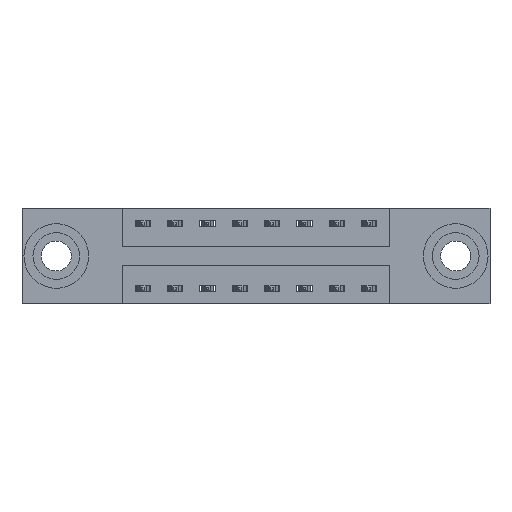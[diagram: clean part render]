
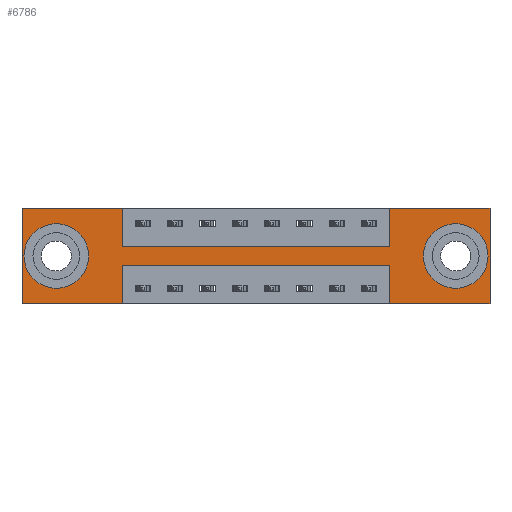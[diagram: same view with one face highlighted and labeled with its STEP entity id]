
A CAD part, front view. The second image highlights one B-rep face of the part: STEP entity #6786.
In plain terms, the highlighted planar face has unit normal (0, -1, 0).
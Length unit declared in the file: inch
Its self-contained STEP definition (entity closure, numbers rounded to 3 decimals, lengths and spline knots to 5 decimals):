
#21 = VECTOR ( 'NONE', #5674, 39.37008 ) ;
#95 = DIRECTION ( 'NONE',  ( 0., 0., 1. ) ) ;
#140 = EDGE_CURVE ( 'NONE', #5483, #7407, #8158, .T. ) ;
#218 = EDGE_CURVE ( 'NONE', #9366, #9716, #7409, .T. ) ;
#443 = FACE_BOUND ( 'NONE', #2200, .T. ) ;
#562 = AXIS2_PLACEMENT_3D ( 'NONE', #6055, #1032, #6862 ) ;
#736 = LINE ( 'NONE', #6050, #8720 ) ;
#753 = CARTESIAN_POINT ( 'NONE',  ( 0.3875, 0., 0. ) ) ;
#939 = AXIS2_PLACEMENT_3D ( 'NONE', #6089, #2746, #8485 ) ;
#1032 = DIRECTION ( 'NONE',  ( 0., 1., 0. ) ) ;
#1037 = CARTESIAN_POINT ( 'NONE',  ( 1.81, 0., 0. ) ) ;
#1053 = CARTESIAN_POINT ( 'NONE',  ( 1.4225, 0., -0.37 ) ) ;
#1063 = CARTESIAN_POINT ( 'NONE',  ( 1.81, 0., 0. ) ) ;
#1160 = ORIENTED_EDGE ( 'NONE', *, *, #9546, .F. ) ;
#1297 = CARTESIAN_POINT ( 'NONE',  ( 0.1325, 0., -0.185 ) ) ;
#1353 = ORIENTED_EDGE ( 'NONE', *, *, #4630, .T. ) ;
#1377 = DIRECTION ( 'NONE',  ( 1., 0., 0. ) ) ;
#1467 = ORIENTED_EDGE ( 'NONE', *, *, #218, .F. ) ;
#1550 = DIRECTION ( 'NONE',  ( 0., 1., 0. ) ) ;
#1577 = ORIENTED_EDGE ( 'NONE', *, *, #9678, .F. ) ;
#1593 = VECTOR ( 'NONE', #7326, 39.37008 ) ;
#1604 = DIRECTION ( 'NONE',  ( 0., 0., -1. ) ) ;
#1704 = AXIS2_PLACEMENT_3D ( 'NONE', #6538, #1550, #7331 ) ;
#1717 = EDGE_CURVE ( 'NONE', #7351, #2289, #8508, .T. ) ;
#1751 = CARTESIAN_POINT ( 'NONE',  ( 1.4225, 0., 0. ) ) ;
#1907 = LINE ( 'NONE', #4998, #10024 ) ;
#1920 = PLANE ( 'NONE',  #939 ) ;
#1961 = VERTEX_POINT ( 'NONE', #7584 ) ;
#1974 = LINE ( 'NONE', #2035, #3958 ) ;
#1984 = LINE ( 'NONE', #4860, #6172 ) ;
#1992 = EDGE_CURVE ( 'NONE', #5678, #4226, #7871, .T. ) ;
#2035 = CARTESIAN_POINT ( 'NONE',  ( 0., 0., -0.37 ) ) ;
#2075 = CIRCLE ( 'NONE', #2267, 0.078 ) ;
#2097 = DIRECTION ( 'NONE',  ( 0., 0., 1. ) ) ;
#2126 = CARTESIAN_POINT ( 'NONE',  ( 0.1325, 0., -0.107 ) ) ;
#2141 = DIRECTION ( 'NONE',  ( 0., 0., 1. ) ) ;
#2200 = EDGE_LOOP ( 'NONE', ( #7179, #1353 ) ) ;
#2224 = EDGE_CURVE ( 'NONE', #4226, #5678, #9817, .T. ) ;
#2250 = AXIS2_PLACEMENT_3D ( 'NONE', #1297, #7099, #2141 ) ;
#2267 = AXIS2_PLACEMENT_3D ( 'NONE', #7399, #2464, #8216 ) ;
#2289 = VERTEX_POINT ( 'NONE', #4767 ) ;
#2301 = CARTESIAN_POINT ( 'NONE',  ( 1.4225, 0., -0.37 ) ) ;
#2464 = DIRECTION ( 'NONE',  ( 0., 1., 0. ) ) ;
#2618 = VECTOR ( 'NONE', #1377, 39.37008 ) ;
#2663 = FACE_BOUND ( 'NONE', #4462, .T. ) ;
#2746 = DIRECTION ( 'NONE',  ( 0., -1., 0. ) ) ;
#2778 = VERTEX_POINT ( 'NONE', #3030 ) ;
#2782 = ORIENTED_EDGE ( 'NONE', *, *, #140, .F. ) ;
#2853 = VERTEX_POINT ( 'NONE', #6460 ) ;
#2868 = DIRECTION ( 'NONE',  ( -1., 0., 0. ) ) ;
#3030 = CARTESIAN_POINT ( 'NONE',  ( 0., 0., 0. ) ) ;
#3063 = CIRCLE ( 'NONE', #1704, 0.078 ) ;
#3576 = CARTESIAN_POINT ( 'NONE',  ( 0.3875, 0., -0.22 ) ) ;
#3653 = ORIENTED_EDGE ( 'NONE', *, *, #10394, .F. ) ;
#3719 = DIRECTION ( 'NONE',  ( 1., 0., 0. ) ) ;
#3753 = CARTESIAN_POINT ( 'NONE',  ( 1.6775, 0., -0.263 ) ) ;
#3958 = VECTOR ( 'NONE', #2868, 39.37008 ) ;
#4028 = ORIENTED_EDGE ( 'NONE', *, *, #9071, .F. ) ;
#4029 = VERTEX_POINT ( 'NONE', #7032 ) ;
#4053 = EDGE_CURVE ( 'NONE', #4668, #7351, #1907, .T. ) ;
#4148 = ORIENTED_EDGE ( 'NONE', *, *, #8516, .F. ) ;
#4226 = VERTEX_POINT ( 'NONE', #9182 ) ;
#4331 = VERTEX_POINT ( 'NONE', #6901 ) ;
#4399 = VERTEX_POINT ( 'NONE', #4602 ) ;
#4462 = EDGE_LOOP ( 'NONE', ( #10114, #4656 ) ) ;
#4602 = CARTESIAN_POINT ( 'NONE',  ( 1.4225, 0., -0.15 ) ) ;
#4630 = EDGE_CURVE ( 'NONE', #5597, #1961, #3063, .T. ) ;
#4656 = ORIENTED_EDGE ( 'NONE', *, *, #2224, .T. ) ;
#4668 = VERTEX_POINT ( 'NONE', #3576 ) ;
#4678 = FACE_OUTER_BOUND ( 'NONE', #5301, .T. ) ;
#4732 = EDGE_CURVE ( 'NONE', #1961, #5597, #2075, .T. ) ;
#4767 = CARTESIAN_POINT ( 'NONE',  ( 0., 0., -0.37 ) ) ;
#4781 = VECTOR ( 'NONE', #1604, 39.37008 ) ;
#4860 = CARTESIAN_POINT ( 'NONE',  ( 0.3875, 0., -0.15 ) ) ;
#4890 = LINE ( 'NONE', #9465, #2618 ) ;
#4978 = EDGE_CURVE ( 'NONE', #7407, #4668, #736, .T. ) ;
#4997 = VECTOR ( 'NONE', #95, 39.37008 ) ;
#4998 = CARTESIAN_POINT ( 'NONE',  ( 0.3875, 0., -0.37 ) ) ;
#5301 = EDGE_LOOP ( 'NONE', ( #6814, #9632, #2782, #1160, #1467, #1577, #3653, #4028, #4148, #9660, #8214, #7216 ) ) ;
#5434 = LINE ( 'NONE', #5449, #7554 ) ;
#5449 = CARTESIAN_POINT ( 'NONE',  ( 0., 0., 0. ) ) ;
#5483 = VERTEX_POINT ( 'NONE', #1053 ) ;
#5586 = EDGE_CURVE ( 'NONE', #2778, #4029, #8228, .T. ) ;
#5597 = VERTEX_POINT ( 'NONE', #3753 ) ;
#5674 = DIRECTION ( 'NONE',  ( -1., 0., 0. ) ) ;
#5678 = VERTEX_POINT ( 'NONE', #2126 ) ;
#6050 = CARTESIAN_POINT ( 'NONE',  ( 0.3875, 0., -0.22 ) ) ;
#6055 = CARTESIAN_POINT ( 'NONE',  ( 0.1325, 0., -0.185 ) ) ;
#6089 = CARTESIAN_POINT ( 'NONE',  ( 0., 0., -0.37 ) ) ;
#6172 = VECTOR ( 'NONE', #9603, 39.37008 ) ;
#6444 = CARTESIAN_POINT ( 'NONE',  ( 0., 0., -0.37 ) ) ;
#6460 = CARTESIAN_POINT ( 'NONE',  ( 1.4225, 0., 0. ) ) ;
#6538 = CARTESIAN_POINT ( 'NONE',  ( 1.6775, 0., -0.185 ) ) ;
#6621 = DIRECTION ( 'NONE',  ( 0., 0., -1. ) ) ;
#6786 = ADVANCED_FACE ( 'NONE', ( #443, #2663, #4678 ), #1920, .T. ) ;
#6814 = ORIENTED_EDGE ( 'NONE', *, *, #4053, .F. ) ;
#6862 = DIRECTION ( 'NONE',  ( 0., 0., 1. ) ) ;
#6901 = CARTESIAN_POINT ( 'NONE',  ( 0.3875, 0., -0.15 ) ) ;
#7032 = CARTESIAN_POINT ( 'NONE',  ( 0.3875, 0., 0. ) ) ;
#7099 = DIRECTION ( 'NONE',  ( 0., 1., 0. ) ) ;
#7170 = LINE ( 'NONE', #753, #4781 ) ;
#7179 = ORIENTED_EDGE ( 'NONE', *, *, #4732, .T. ) ;
#7216 = ORIENTED_EDGE ( 'NONE', *, *, #1717, .F. ) ;
#7326 = DIRECTION ( 'NONE',  ( 0., 0., 1. ) ) ;
#7331 = DIRECTION ( 'NONE',  ( 0., 0., -1. ) ) ;
#7351 = VERTEX_POINT ( 'NONE', #8179 ) ;
#7399 = CARTESIAN_POINT ( 'NONE',  ( 1.6775, 0., -0.185 ) ) ;
#7407 = VERTEX_POINT ( 'NONE', #9034 ) ;
#7409 = LINE ( 'NONE', #1063, #9736 ) ;
#7554 = VECTOR ( 'NONE', #2097, 39.37008 ) ;
#7584 = CARTESIAN_POINT ( 'NONE',  ( 1.6775, 0., -0.107 ) ) ;
#7871 = CIRCLE ( 'NONE', #562, 0.078 ) ;
#7995 = CARTESIAN_POINT ( 'NONE',  ( 1.81, 0., -0.37 ) ) ;
#8054 = DIRECTION ( 'NONE',  ( 0., 0., -1. ) ) ;
#8158 = LINE ( 'NONE', #2301, #1593 ) ;
#8179 = CARTESIAN_POINT ( 'NONE',  ( 0.3875, 0., -0.37 ) ) ;
#8214 = ORIENTED_EDGE ( 'NONE', *, *, #8268, .F. ) ;
#8216 = DIRECTION ( 'NONE',  ( 0., 0., -1. ) ) ;
#8228 = LINE ( 'NONE', #9356, #9552 ) ;
#8268 = EDGE_CURVE ( 'NONE', #2289, #2778, #5434, .T. ) ;
#8485 = DIRECTION ( 'NONE',  ( 0., 0., -1. ) ) ;
#8508 = LINE ( 'NONE', #6444, #21 ) ;
#8516 = EDGE_CURVE ( 'NONE', #4029, #4331, #7170, .T. ) ;
#8720 = VECTOR ( 'NONE', #9231, 39.37008 ) ;
#9034 = CARTESIAN_POINT ( 'NONE',  ( 1.4225, 0., -0.22 ) ) ;
#9071 = EDGE_CURVE ( 'NONE', #4331, #4399, #1984, .T. ) ;
#9182 = CARTESIAN_POINT ( 'NONE',  ( 0.1325, 0., -0.263 ) ) ;
#9231 = DIRECTION ( 'NONE',  ( -1., 0., 0. ) ) ;
#9237 = LINE ( 'NONE', #1751, #4997 ) ;
#9356 = CARTESIAN_POINT ( 'NONE',  ( 0., 0., 0. ) ) ;
#9366 = VERTEX_POINT ( 'NONE', #1037 ) ;
#9465 = CARTESIAN_POINT ( 'NONE',  ( 0., 0., 0. ) ) ;
#9546 = EDGE_CURVE ( 'NONE', #9716, #5483, #1974, .T. ) ;
#9552 = VECTOR ( 'NONE', #3719, 39.37008 ) ;
#9603 = DIRECTION ( 'NONE',  ( 1., 0., 0. ) ) ;
#9632 = ORIENTED_EDGE ( 'NONE', *, *, #4978, .F. ) ;
#9660 = ORIENTED_EDGE ( 'NONE', *, *, #5586, .F. ) ;
#9678 = EDGE_CURVE ( 'NONE', #2853, #9366, #4890, .T. ) ;
#9716 = VERTEX_POINT ( 'NONE', #7995 ) ;
#9736 = VECTOR ( 'NONE', #8054, 39.37008 ) ;
#9817 = CIRCLE ( 'NONE', #2250, 0.078 ) ;
#10024 = VECTOR ( 'NONE', #6621, 39.37008 ) ;
#10114 = ORIENTED_EDGE ( 'NONE', *, *, #1992, .T. ) ;
#10394 = EDGE_CURVE ( 'NONE', #4399, #2853, #9237, .T. ) ;
